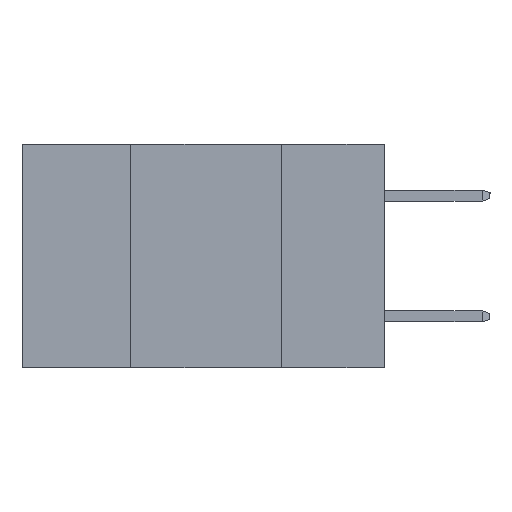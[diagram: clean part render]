
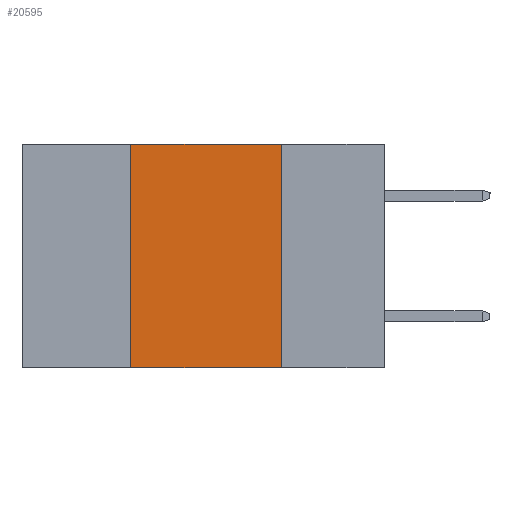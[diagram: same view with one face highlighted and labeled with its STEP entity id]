
A CAD part, left-side view. The second image highlights one B-rep face of the part: STEP entity #20595.
In plain terms, the highlighted planar face has unit normal (-1, 0, 0).
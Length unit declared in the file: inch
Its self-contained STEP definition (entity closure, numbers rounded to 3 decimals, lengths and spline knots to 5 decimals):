
#1122 = DIRECTION ( 'NONE',  ( 0., -1., 0. ) ) ;
#1603 = ORIENTED_EDGE ( 'NONE', *, *, #16503, .F. ) ;
#1794 = LINE ( 'NONE', #5455, #6893 ) ;
#2691 = ORIENTED_EDGE ( 'NONE', *, *, #16572, .F. ) ;
#2750 = VERTEX_POINT ( 'NONE', #9071 ) ;
#2756 = CARTESIAN_POINT ( 'NONE',  ( 0., 0.6, -0.37 ) ) ;
#3682 = CARTESIAN_POINT ( 'NONE',  ( 0., 0.42, -0.37 ) ) ;
#3878 = VECTOR ( 'NONE', #20013, 39.37008 ) ;
#3930 = AXIS2_PLACEMENT_3D ( 'NONE', #15890, #4938, #5173 ) ;
#4697 = VECTOR ( 'NONE', #1122, 39.37008 ) ;
#4938 = DIRECTION ( 'NONE',  ( 1., 0., 0. ) ) ;
#5173 = DIRECTION ( 'NONE',  ( 0., 0., -1. ) ) ;
#5455 = CARTESIAN_POINT ( 'NONE',  ( 0., 0.6, 0. ) ) ;
#5758 = VECTOR ( 'NONE', #14294, 39.37008 ) ;
#6727 = FACE_OUTER_BOUND ( 'NONE', #23264, .T. ) ;
#6893 = VECTOR ( 'NONE', #21487, 39.37008 ) ;
#9071 = CARTESIAN_POINT ( 'NONE',  ( 0., 0.17, -0.37 ) ) ;
#10584 = CARTESIAN_POINT ( 'NONE',  ( 0., 0.17, -0.37 ) ) ;
#10591 = VERTEX_POINT ( 'NONE', #12001 ) ;
#11029 = PLANE ( 'NONE',  #3930 ) ;
#12001 = CARTESIAN_POINT ( 'NONE',  ( 0., 0.42, -0.37 ) ) ;
#12467 = LINE ( 'NONE', #10584, #3878 ) ;
#13529 = VERTEX_POINT ( 'NONE', #14525 ) ;
#14294 = DIRECTION ( 'NONE',  ( 0., 0., 1. ) ) ;
#14525 = CARTESIAN_POINT ( 'NONE',  ( 0., 0.17, 0. ) ) ;
#14631 = ORIENTED_EDGE ( 'NONE', *, *, #18812, .F. ) ;
#15260 = LINE ( 'NONE', #2756, #4697 ) ;
#15890 = CARTESIAN_POINT ( 'NONE',  ( 0., 0.6, 0. ) ) ;
#16503 = EDGE_CURVE ( 'NONE', #10591, #16937, #18073, .T. ) ;
#16572 = EDGE_CURVE ( 'NONE', #16937, #13529, #1794, .T. ) ;
#16937 = VERTEX_POINT ( 'NONE', #22650 ) ;
#18073 = LINE ( 'NONE', #3682, #5758 ) ;
#18812 = EDGE_CURVE ( 'NONE', #13529, #2750, #12467, .T. ) ;
#20013 = DIRECTION ( 'NONE',  ( 0., 0., -1. ) ) ;
#20595 = ADVANCED_FACE ( 'NONE', ( #6727 ), #11029, .F. ) ;
#20782 = EDGE_CURVE ( 'NONE', #10591, #2750, #15260, .T. ) ;
#21487 = DIRECTION ( 'NONE',  ( 0., -1., 0. ) ) ;
#22650 = CARTESIAN_POINT ( 'NONE',  ( 0., 0.42, 0. ) ) ;
#23128 = ORIENTED_EDGE ( 'NONE', *, *, #20782, .T. ) ;
#23264 = EDGE_LOOP ( 'NONE', ( #14631, #2691, #1603, #23128 ) ) ;
